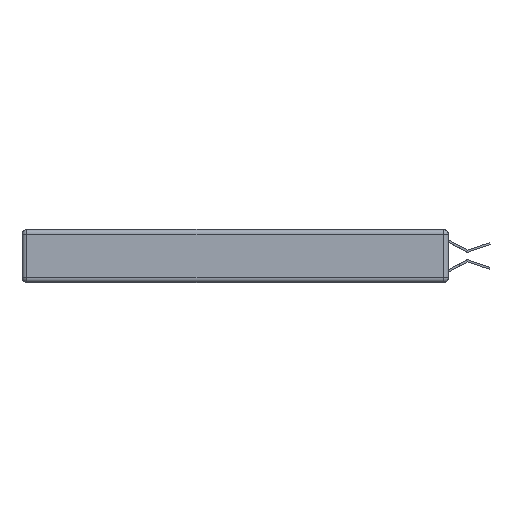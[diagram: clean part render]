
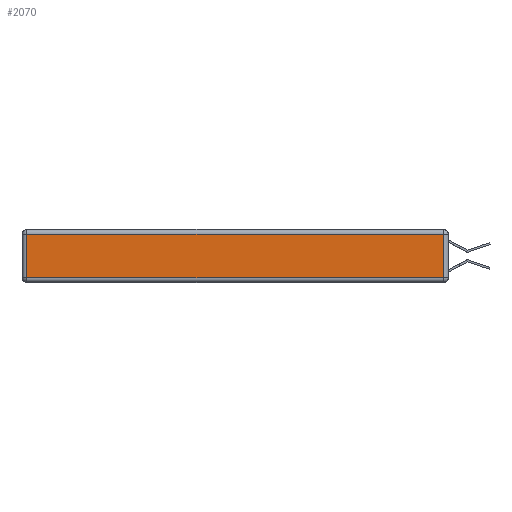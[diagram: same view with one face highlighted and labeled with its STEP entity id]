
A CAD part, left-side view. The second image highlights one B-rep face of the part: STEP entity #2070.
In plain terms, the highlighted planar face has unit normal (-1, 0, 0).
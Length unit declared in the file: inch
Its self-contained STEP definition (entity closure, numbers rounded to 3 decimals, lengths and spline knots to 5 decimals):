
#1271 = DIRECTION ( 'NONE',  ( 0., 0., 1. ) ) ;
#1900 = VERTEX_POINT ( 'NONE', #4015 ) ;
#2070 = ADVANCED_FACE ( 'NONE', ( #8147 ), #4198, .T. ) ;
#2564 = EDGE_CURVE ( 'NONE', #16285, #4114, #14824, .T. ) ;
#2590 = VECTOR ( 'NONE', #14281, 39.37008 ) ;
#3127 = CARTESIAN_POINT ( 'NONE',  ( 0., 0., -0.313 ) ) ;
#3296 = VERTEX_POINT ( 'NONE', #16207 ) ;
#3861 = EDGE_CURVE ( 'NONE', #3296, #1900, #5037, .T. ) ;
#4015 = CARTESIAN_POINT ( 'NONE',  ( 0., 0.03, -0.313 ) ) ;
#4114 = VERTEX_POINT ( 'NONE', #19514 ) ;
#4198 = PLANE ( 'NONE',  #16040 ) ;
#4353 = LINE ( 'NONE', #15666, #8877 ) ;
#4486 = CARTESIAN_POINT ( 'NONE',  ( 0., 0., -0.343 ) ) ;
#4736 = DIRECTION ( 'NONE',  ( 0., 0., -1. ) ) ;
#5037 = LINE ( 'NONE', #3127, #9318 ) ;
#8147 = FACE_OUTER_BOUND ( 'NONE', #19650, .T. ) ;
#8149 = CARTESIAN_POINT ( 'NONE',  ( 0., 2.75, -0.03 ) ) ;
#8823 = ORIENTED_EDGE ( 'NONE', *, *, #2564, .T. ) ;
#8877 = VECTOR ( 'NONE', #1271, 39.37008 ) ;
#9253 = DIRECTION ( 'NONE',  ( -1., 0., 0. ) ) ;
#9318 = VECTOR ( 'NONE', #11075, 39.37008 ) ;
#9559 = CARTESIAN_POINT ( 'NONE',  ( 0., 0.03, -0.03 ) ) ;
#11055 = ORIENTED_EDGE ( 'NONE', *, *, #3861, .T. ) ;
#11075 = DIRECTION ( 'NONE',  ( 0., -1., 0. ) ) ;
#11989 = EDGE_CURVE ( 'NONE', #1900, #16285, #4353, .T. ) ;
#12107 = ORIENTED_EDGE ( 'NONE', *, *, #13169, .T. ) ;
#13169 = EDGE_CURVE ( 'NONE', #4114, #3296, #16651, .T. ) ;
#14281 = DIRECTION ( 'NONE',  ( 0., 1., 0. ) ) ;
#14824 = LINE ( 'NONE', #8149, #2590 ) ;
#15425 = VECTOR ( 'NONE', #4736, 39.37008 ) ;
#15666 = CARTESIAN_POINT ( 'NONE',  ( 0., 0.03, -0.343 ) ) ;
#15919 = CARTESIAN_POINT ( 'NONE',  ( 0., 2.72, -0.343 ) ) ;
#16040 = AXIS2_PLACEMENT_3D ( 'NONE', #4486, #9253, #20452 ) ;
#16207 = CARTESIAN_POINT ( 'NONE',  ( 0., 2.72, -0.313 ) ) ;
#16285 = VERTEX_POINT ( 'NONE', #9559 ) ;
#16651 = LINE ( 'NONE', #15919, #15425 ) ;
#19514 = CARTESIAN_POINT ( 'NONE',  ( 0., 2.72, -0.03 ) ) ;
#19650 = EDGE_LOOP ( 'NONE', ( #11055, #20247, #8823, #12107 ) ) ;
#20247 = ORIENTED_EDGE ( 'NONE', *, *, #11989, .T. ) ;
#20452 = DIRECTION ( 'NONE',  ( 0., 0., 1. ) ) ;
